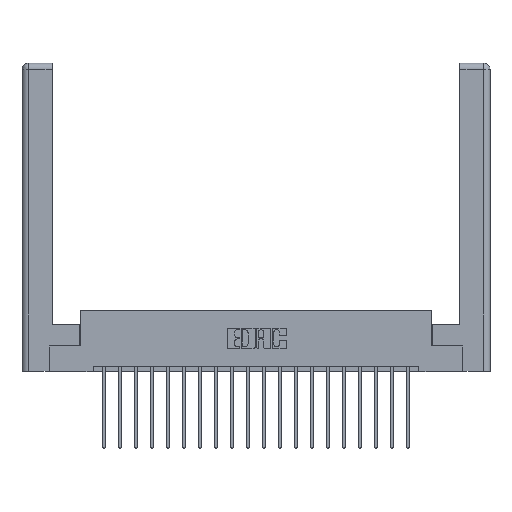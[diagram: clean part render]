
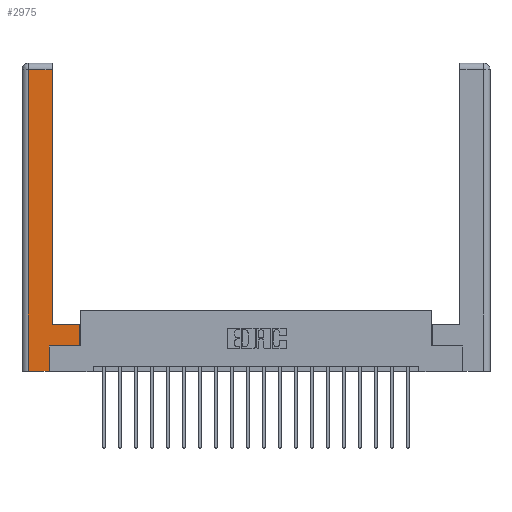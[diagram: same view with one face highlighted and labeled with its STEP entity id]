
A CAD part, top view. The second image highlights one B-rep face of the part: STEP entity #2975.
In plain terms, the highlighted planar face has unit normal (0, 0, 1).
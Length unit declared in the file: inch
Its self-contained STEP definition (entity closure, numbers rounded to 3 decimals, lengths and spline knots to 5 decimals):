
#1106 = VECTOR ( 'NONE', #10952, 39.37008 ) ;
#1251 = CARTESIAN_POINT ( 'NONE',  ( 0.565, 0.245, 0. ) ) ;
#2058 = AXIS2_PLACEMENT_3D ( 'NONE', #19104, #12630, #6679 ) ;
#2338 = CARTESIAN_POINT ( 'NONE',  ( 0.295, 2.94, 0. ) ) ;
#2455 = EDGE_CURVE ( 'NONE', #3114, #18349, #12250, .T. ) ;
#2734 = CARTESIAN_POINT ( 'NONE',  ( 0.0615, 2.94, 0. ) ) ;
#2975 = ADVANCED_FACE ( 'NONE', ( #17030 ), #6132, .F. ) ;
#3006 = DIRECTION ( 'NONE',  ( 0., 1., 0. ) ) ;
#3114 = VERTEX_POINT ( 'NONE', #3474 ) ;
#3474 = CARTESIAN_POINT ( 'NONE',  ( 0.565, 0.45, 0. ) ) ;
#3797 = DIRECTION ( 'NONE',  ( 0., 1., 0. ) ) ;
#4299 = VERTEX_POINT ( 'NONE', #7440 ) ;
#4318 = ORIENTED_EDGE ( 'NONE', *, *, #12685, .T. ) ;
#4530 = CARTESIAN_POINT ( 'NONE',  ( 0.0615, 2.94, 0. ) ) ;
#5238 = VECTOR ( 'NONE', #3006, 39.37008 ) ;
#6132 = PLANE ( 'NONE',  #2058 ) ;
#6679 = DIRECTION ( 'NONE',  ( -1., 0., 0. ) ) ;
#6727 = ORIENTED_EDGE ( 'NONE', *, *, #9570, .T. ) ;
#7341 = DIRECTION ( 'NONE',  ( 0., 1., 0. ) ) ;
#7440 = CARTESIAN_POINT ( 'NONE',  ( 0.0615, 0., 0. ) ) ;
#7694 = VECTOR ( 'NONE', #3797, 39.37008 ) ;
#7733 = EDGE_CURVE ( 'NONE', #11039, #11371, #11334, .T. ) ;
#7865 = VECTOR ( 'NONE', #11296, 39.37008 ) ;
#7958 = EDGE_CURVE ( 'NONE', #18349, #11039, #18691, .T. ) ;
#8140 = CARTESIAN_POINT ( 'NONE',  ( 0.265, 0.245, 0. ) ) ;
#8462 = EDGE_CURVE ( 'NONE', #4299, #17456, #10806, .T. ) ;
#9078 = CARTESIAN_POINT ( 'NONE',  ( 0.265, 0.245, 0. ) ) ;
#9570 = EDGE_CURVE ( 'NONE', #18607, #3114, #18876, .T. ) ;
#9750 = ORIENTED_EDGE ( 'NONE', *, *, #8462, .T. ) ;
#10489 = CARTESIAN_POINT ( 'NONE',  ( 0.565, 0.45, 0. ) ) ;
#10806 = LINE ( 'NONE', #20732, #19179 ) ;
#10835 = DIRECTION ( 'NONE',  ( -1., 0., 0. ) ) ;
#10952 = DIRECTION ( 'NONE',  ( -1., 0., 0. ) ) ;
#11039 = VERTEX_POINT ( 'NONE', #2338 ) ;
#11088 = VECTOR ( 'NONE', #10835, 39.37008 ) ;
#11150 = CARTESIAN_POINT ( 'NONE',  ( 0.0615, 0., 0. ) ) ;
#11168 = CARTESIAN_POINT ( 'NONE',  ( 0.295, 3., 0. ) ) ;
#11296 = DIRECTION ( 'NONE',  ( 0., -1., 0. ) ) ;
#11334 = LINE ( 'NONE', #2734, #11088 ) ;
#11371 = VERTEX_POINT ( 'NONE', #4530 ) ;
#12250 = LINE ( 'NONE', #20712, #1106 ) ;
#12568 = ORIENTED_EDGE ( 'NONE', *, *, #15161, .T. ) ;
#12630 = DIRECTION ( 'NONE',  ( 0., 0., -1. ) ) ;
#12685 = EDGE_CURVE ( 'NONE', #11371, #4299, #18261, .T. ) ;
#13902 = CARTESIAN_POINT ( 'NONE',  ( 0.265, 0., 0. ) ) ;
#14462 = VECTOR ( 'NONE', #7341, 39.37008 ) ;
#14573 = DIRECTION ( 'NONE',  ( 1., 0., 0. ) ) ;
#15161 = EDGE_CURVE ( 'NONE', #20036, #18607, #19166, .T. ) ;
#15487 = ORIENTED_EDGE ( 'NONE', *, *, #7733, .T. ) ;
#16275 = LINE ( 'NONE', #9078, #14462 ) ;
#16471 = EDGE_LOOP ( 'NONE', ( #17576, #15487, #4318, #9750, #18509, #12568, #6727, #20220 ) ) ;
#17030 = FACE_OUTER_BOUND ( 'NONE', #16471, .T. ) ;
#17456 = VERTEX_POINT ( 'NONE', #13902 ) ;
#17576 = ORIENTED_EDGE ( 'NONE', *, *, #7958, .T. ) ;
#18261 = LINE ( 'NONE', #11150, #7865 ) ;
#18349 = VERTEX_POINT ( 'NONE', #18715 ) ;
#18509 = ORIENTED_EDGE ( 'NONE', *, *, #20389, .T. ) ;
#18607 = VERTEX_POINT ( 'NONE', #1251 ) ;
#18691 = LINE ( 'NONE', #11168, #5238 ) ;
#18715 = CARTESIAN_POINT ( 'NONE',  ( 0.295, 0.45, 0. ) ) ;
#18876 = LINE ( 'NONE', #10489, #7694 ) ;
#19104 = CARTESIAN_POINT ( 'NONE',  ( 0., 0., 0. ) ) ;
#19166 = LINE ( 'NONE', #19495, #20200 ) ;
#19179 = VECTOR ( 'NONE', #20648, 39.37008 ) ;
#19495 = CARTESIAN_POINT ( 'NONE',  ( 0.565, 0.245, 0. ) ) ;
#20036 = VERTEX_POINT ( 'NONE', #8140 ) ;
#20200 = VECTOR ( 'NONE', #14573, 39.37008 ) ;
#20220 = ORIENTED_EDGE ( 'NONE', *, *, #2455, .T. ) ;
#20389 = EDGE_CURVE ( 'NONE', #17456, #20036, #16275, .T. ) ;
#20648 = DIRECTION ( 'NONE',  ( 1., 0., 0. ) ) ;
#20712 = CARTESIAN_POINT ( 'NONE',  ( 0.295, 0.45, 0. ) ) ;
#20732 = CARTESIAN_POINT ( 'NONE',  ( 0.265, 0., 0. ) ) ;
